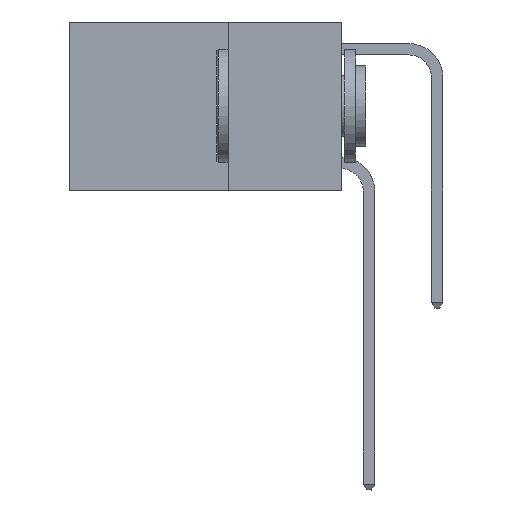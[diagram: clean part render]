
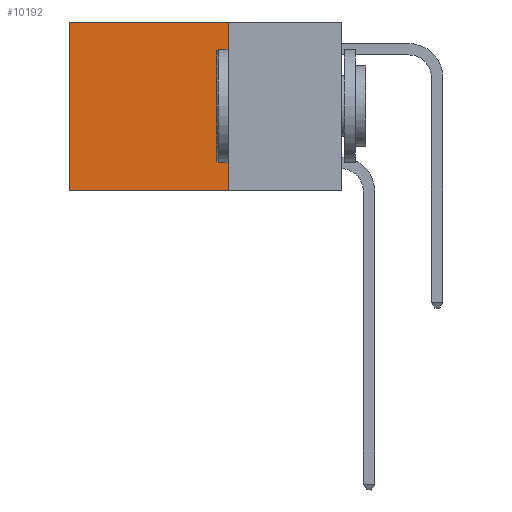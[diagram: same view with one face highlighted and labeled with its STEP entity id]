
A CAD part, left-side view. The second image highlights one B-rep face of the part: STEP entity #10192.
In plain terms, the highlighted planar face has unit normal (-1, 0, 0).
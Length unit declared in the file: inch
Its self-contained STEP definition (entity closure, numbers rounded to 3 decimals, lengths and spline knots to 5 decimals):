
#565 = VECTOR ( 'NONE', #23600, 39.37008 ) ;
#3823 = CARTESIAN_POINT ( 'NONE',  ( 0.2625, 0.25, 0. ) ) ;
#3868 = CARTESIAN_POINT ( 'NONE',  ( 0.2625, 0.6, -0.37 ) ) ;
#4004 = CARTESIAN_POINT ( 'NONE',  ( 0.2625, 0.25, 0. ) ) ;
#4868 = EDGE_CURVE ( 'NONE', #21188, #15150, #18484, .T. ) ;
#5689 = LINE ( 'NONE', #27704, #28373 ) ;
#6301 = DIRECTION ( 'NONE',  ( 0., 0., -1. ) ) ;
#6342 = FACE_OUTER_BOUND ( 'NONE', #23638, .T. ) ;
#8647 = DIRECTION ( 'NONE',  ( 0., 1., 0. ) ) ;
#8803 = LINE ( 'NONE', #15960, #565 ) ;
#8998 = DIRECTION ( 'NONE',  ( 1., 0., 0. ) ) ;
#9430 = EDGE_CURVE ( 'NONE', #24742, #24876, #5689, .T. ) ;
#9610 = ORIENTED_EDGE ( 'NONE', *, *, #17674, .F. ) ;
#10192 = ADVANCED_FACE ( 'NONE', ( #6342 ), #29785, .F. ) ;
#10304 = ORIENTED_EDGE ( 'NONE', *, *, #9430, .F. ) ;
#11933 = CARTESIAN_POINT ( 'NONE',  ( 0.2625, 0.6, 0. ) ) ;
#12572 = EDGE_CURVE ( 'NONE', #24742, #21188, #30479, .T. ) ;
#12798 = VECTOR ( 'NONE', #8647, 39.37008 ) ;
#13886 = AXIS2_PLACEMENT_3D ( 'NONE', #4004, #8998, #15856 ) ;
#14273 = DIRECTION ( 'NONE',  ( 0., 0., -1. ) ) ;
#15150 = VERTEX_POINT ( 'NONE', #3868 ) ;
#15856 = DIRECTION ( 'NONE',  ( 0., 0., -1. ) ) ;
#15960 = CARTESIAN_POINT ( 'NONE',  ( 0.2625, 0.25, -0.37 ) ) ;
#17674 = EDGE_CURVE ( 'NONE', #24876, #15150, #8803, .T. ) ;
#17855 = ORIENTED_EDGE ( 'NONE', *, *, #12572, .T. ) ;
#18484 = LINE ( 'NONE', #11933, #20774 ) ;
#19073 = ORIENTED_EDGE ( 'NONE', *, *, #4868, .T. ) ;
#20774 = VECTOR ( 'NONE', #14273, 39.37008 ) ;
#21188 = VERTEX_POINT ( 'NONE', #28256 ) ;
#23455 = CARTESIAN_POINT ( 'NONE',  ( 0.2625, 0.25, -0.37 ) ) ;
#23600 = DIRECTION ( 'NONE',  ( 0., 1., 0. ) ) ;
#23638 = EDGE_LOOP ( 'NONE', ( #19073, #9610, #10304, #17855 ) ) ;
#24742 = VERTEX_POINT ( 'NONE', #25046 ) ;
#24876 = VERTEX_POINT ( 'NONE', #23455 ) ;
#25046 = CARTESIAN_POINT ( 'NONE',  ( 0.2625, 0.25, 0. ) ) ;
#27704 = CARTESIAN_POINT ( 'NONE',  ( 0.2625, 0.25, 0. ) ) ;
#28256 = CARTESIAN_POINT ( 'NONE',  ( 0.2625, 0.6, 0. ) ) ;
#28373 = VECTOR ( 'NONE', #6301, 39.37008 ) ;
#29785 = PLANE ( 'NONE',  #13886 ) ;
#30479 = LINE ( 'NONE', #3823, #12798 ) ;
